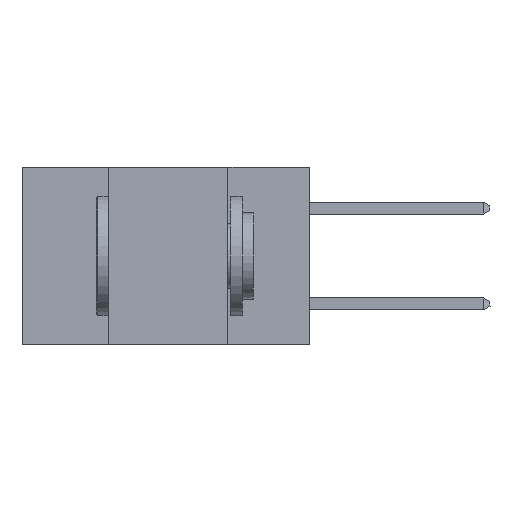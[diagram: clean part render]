
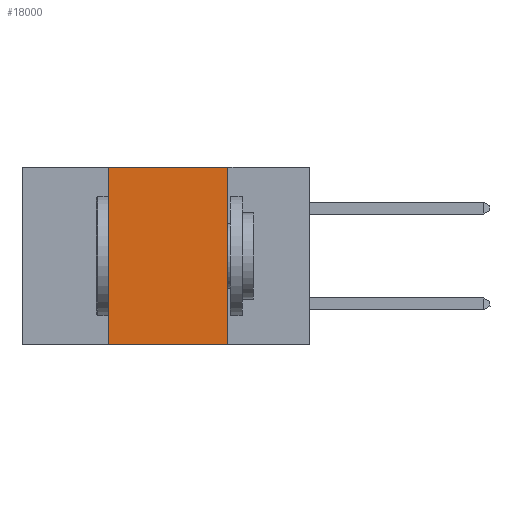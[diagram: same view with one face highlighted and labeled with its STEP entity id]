
A CAD part, left-side view. The second image highlights one B-rep face of the part: STEP entity #18000.
In plain terms, the highlighted planar face has unit normal (-1, 0, 0).
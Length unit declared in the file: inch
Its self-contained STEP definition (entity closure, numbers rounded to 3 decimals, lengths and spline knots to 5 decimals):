
#1318 = CARTESIAN_POINT ( 'NONE',  ( 0., 0.6, -0.37 ) ) ;
#3241 = LINE ( 'NONE', #1318, #16386 ) ;
#3484 = EDGE_LOOP ( 'NONE', ( #19937, #14532, #10023, #10060 ) ) ;
#3828 = CARTESIAN_POINT ( 'NONE',  ( 0., 0.17, 0. ) ) ;
#4230 = PLANE ( 'NONE',  #17414 ) ;
#5758 = FACE_OUTER_BOUND ( 'NONE', #3484, .T. ) ;
#7763 = EDGE_CURVE ( 'NONE', #20915, #15414, #14893, .T. ) ;
#8792 = LINE ( 'NONE', #17799, #17533 ) ;
#9153 = DIRECTION ( 'NONE',  ( 1., 0., 0. ) ) ;
#9431 = CARTESIAN_POINT ( 'NONE',  ( 0., 0.17, -0.37 ) ) ;
#9504 = VECTOR ( 'NONE', #13495, 39.37008 ) ;
#9625 = DIRECTION ( 'NONE',  ( 0., -1., 0. ) ) ;
#10023 = ORIENTED_EDGE ( 'NONE', *, *, #14406, .F. ) ;
#10060 = ORIENTED_EDGE ( 'NONE', *, *, #15502, .T. ) ;
#10549 = VECTOR ( 'NONE', #19490, 39.37008 ) ;
#11376 = DIRECTION ( 'NONE',  ( 0., -1., 0. ) ) ;
#12988 = CARTESIAN_POINT ( 'NONE',  ( 0., 0.17, 0. ) ) ;
#13495 = DIRECTION ( 'NONE',  ( 0., 0., 1. ) ) ;
#14406 = EDGE_CURVE ( 'NONE', #14593, #17234, #18236, .T. ) ;
#14532 = ORIENTED_EDGE ( 'NONE', *, *, #19471, .F. ) ;
#14593 = VERTEX_POINT ( 'NONE', #18875 ) ;
#14893 = LINE ( 'NONE', #12988, #10549 ) ;
#15414 = VERTEX_POINT ( 'NONE', #9431 ) ;
#15502 = EDGE_CURVE ( 'NONE', #14593, #15414, #3241, .T. ) ;
#16386 = VECTOR ( 'NONE', #11376, 39.37008 ) ;
#17234 = VERTEX_POINT ( 'NONE', #20074 ) ;
#17414 = AXIS2_PLACEMENT_3D ( 'NONE', #19000, #9153, #20613 ) ;
#17533 = VECTOR ( 'NONE', #9625, 39.37008 ) ;
#17799 = CARTESIAN_POINT ( 'NONE',  ( 0., 0.6, 0. ) ) ;
#18000 = ADVANCED_FACE ( 'NONE', ( #5758 ), #4230, .F. ) ;
#18236 = LINE ( 'NONE', #18302, #9504 ) ;
#18302 = CARTESIAN_POINT ( 'NONE',  ( 0., 0.42, 0. ) ) ;
#18875 = CARTESIAN_POINT ( 'NONE',  ( 0., 0.42, -0.37 ) ) ;
#19000 = CARTESIAN_POINT ( 'NONE',  ( 0., 0.6, 0. ) ) ;
#19471 = EDGE_CURVE ( 'NONE', #17234, #20915, #8792, .T. ) ;
#19490 = DIRECTION ( 'NONE',  ( 0., 0., -1. ) ) ;
#19937 = ORIENTED_EDGE ( 'NONE', *, *, #7763, .F. ) ;
#20074 = CARTESIAN_POINT ( 'NONE',  ( 0., 0.42, 0. ) ) ;
#20613 = DIRECTION ( 'NONE',  ( 0., 0., -1. ) ) ;
#20915 = VERTEX_POINT ( 'NONE', #3828 ) ;
